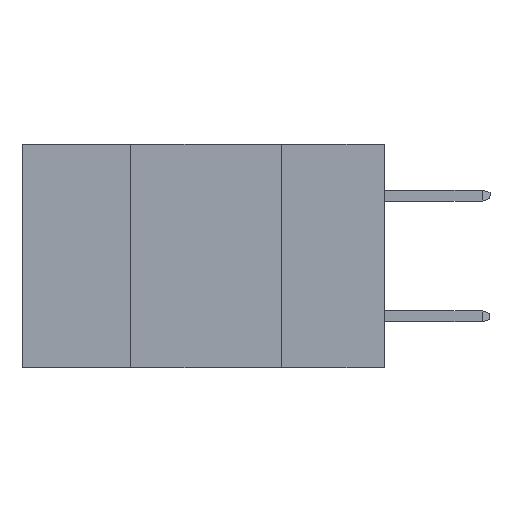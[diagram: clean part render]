
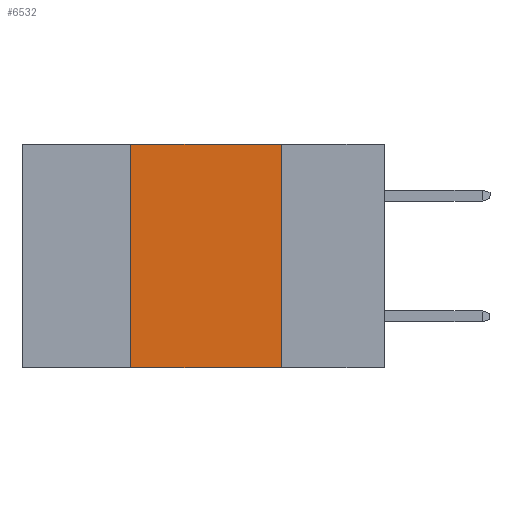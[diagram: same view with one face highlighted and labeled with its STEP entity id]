
A CAD part, left-side view. The second image highlights one B-rep face of the part: STEP entity #6532.
In plain terms, the highlighted planar face has unit normal (-1, 0, 0).
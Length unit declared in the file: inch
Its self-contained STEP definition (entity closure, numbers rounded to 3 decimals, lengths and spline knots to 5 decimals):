
#670 = VECTOR ( 'NONE', #8737, 39.37008 ) ;
#1585 = ORIENTED_EDGE ( 'NONE', *, *, #5232, .F. ) ;
#2162 = LINE ( 'NONE', #5217, #8565 ) ;
#2224 = CARTESIAN_POINT ( 'NONE',  ( 0., 0.6, 0. ) ) ;
#2268 = DIRECTION ( 'NONE',  ( 0., 0., -1. ) ) ;
#2948 = DIRECTION ( 'NONE',  ( 0., 0., 1. ) ) ;
#3140 = EDGE_CURVE ( 'NONE', #4203, #7881, #6511, .T. ) ;
#3278 = CARTESIAN_POINT ( 'NONE',  ( 0., 0.6, -0.37 ) ) ;
#3375 = CARTESIAN_POINT ( 'NONE',  ( 0., 0.17, -0.37 ) ) ;
#3524 = VERTEX_POINT ( 'NONE', #5887 ) ;
#4187 = DIRECTION ( 'NONE',  ( 0., -1., 0. ) ) ;
#4203 = VERTEX_POINT ( 'NONE', #6652 ) ;
#4217 = PLANE ( 'NONE',  #7334 ) ;
#5217 = CARTESIAN_POINT ( 'NONE',  ( 0., 0.42, -0.37 ) ) ;
#5232 = EDGE_CURVE ( 'NONE', #6325, #4203, #9589, .T. ) ;
#5259 = VECTOR ( 'NONE', #9026, 39.37008 ) ;
#5286 = DIRECTION ( 'NONE',  ( 1., 0., 0. ) ) ;
#5593 = ORIENTED_EDGE ( 'NONE', *, *, #3140, .F. ) ;
#5744 = CARTESIAN_POINT ( 'NONE',  ( 0., 0.42, 0. ) ) ;
#5861 = EDGE_CURVE ( 'NONE', #3524, #6325, #2162, .T. ) ;
#5885 = EDGE_CURVE ( 'NONE', #3524, #7881, #7933, .T. ) ;
#5887 = CARTESIAN_POINT ( 'NONE',  ( 0., 0.42, -0.37 ) ) ;
#6325 = VERTEX_POINT ( 'NONE', #5744 ) ;
#6357 = ORIENTED_EDGE ( 'NONE', *, *, #5861, .F. ) ;
#6511 = LINE ( 'NONE', #3375, #670 ) ;
#6532 = ADVANCED_FACE ( 'NONE', ( #8069 ), #4217, .F. ) ;
#6652 = CARTESIAN_POINT ( 'NONE',  ( 0., 0.17, 0. ) ) ;
#7257 = CARTESIAN_POINT ( 'NONE',  ( 0., 0.6, 0. ) ) ;
#7334 = AXIS2_PLACEMENT_3D ( 'NONE', #2224, #5286, #2268 ) ;
#7881 = VERTEX_POINT ( 'NONE', #9656 ) ;
#7933 = LINE ( 'NONE', #3278, #8536 ) ;
#8013 = ORIENTED_EDGE ( 'NONE', *, *, #5885, .T. ) ;
#8069 = FACE_OUTER_BOUND ( 'NONE', #9229, .T. ) ;
#8536 = VECTOR ( 'NONE', #4187, 39.37008 ) ;
#8565 = VECTOR ( 'NONE', #2948, 39.37008 ) ;
#8737 = DIRECTION ( 'NONE',  ( 0., 0., -1. ) ) ;
#9026 = DIRECTION ( 'NONE',  ( 0., -1., 0. ) ) ;
#9229 = EDGE_LOOP ( 'NONE', ( #5593, #1585, #6357, #8013 ) ) ;
#9589 = LINE ( 'NONE', #7257, #5259 ) ;
#9656 = CARTESIAN_POINT ( 'NONE',  ( 0., 0.17, -0.37 ) ) ;
